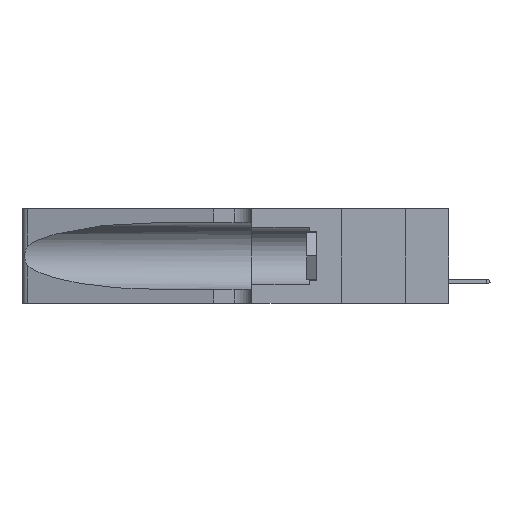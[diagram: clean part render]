
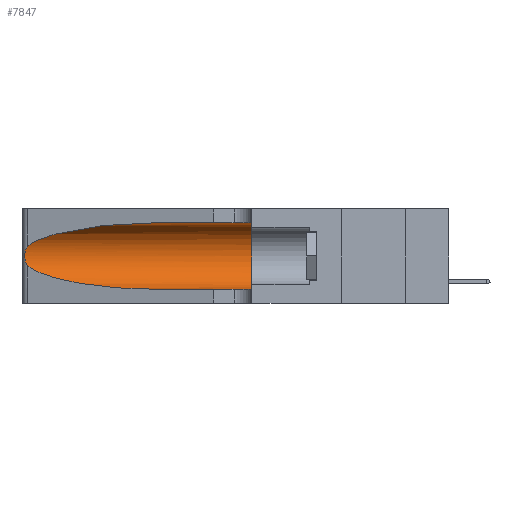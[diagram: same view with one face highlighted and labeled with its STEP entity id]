
A CAD part, left-side view. The second image highlights one B-rep face of the part: STEP entity #7847.
In plain terms, the highlighted cylindrical face has radius 3.308 mm (diameter 6.617 mm), a partial arc.
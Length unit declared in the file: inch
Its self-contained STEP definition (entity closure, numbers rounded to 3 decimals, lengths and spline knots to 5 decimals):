
#718 = LINE ( 'NONE', #38423, #27202 ) ;
#2604 = B_SPLINE_CURVE_WITH_KNOTS ( 'NONE', 3,
 ( #21177, #10785, #30940, #25056, #38808, #35554, #11384, #17910, #32139, #31533, #13188, #12435, #8761, #18988 ),
 .UNSPECIFIED., .F., .F.,
 ( 4, 2, 2, 2, 2, 2, 4 ),
 ( 0., 0.00027, 0.00053, 0.00107, 0.0016, 0.00187, 0.00214 ),
 .UNSPECIFIED. ) ;
#3382 = LINE ( 'NONE', #12412, #14491 ) ;
#3507 = CIRCLE ( 'NONE', #7570, 0.13025 ) ;
#3536 = DIRECTION ( 'NONE',  ( 0., 0., -1. ) ) ;
#4302 = CARTESIAN_POINT ( 'NONE',  ( 0.1305, 0.35, 0.185 ) ) ;
#5955 = CYLINDRICAL_SURFACE ( 'NONE', #28047, 0.13025 ) ;
#7346 = CARTESIAN_POINT ( 'NONE',  ( 0.25487, 1.22718, 0.22369 ) ) ;
#7570 = AXIS2_PLACEMENT_3D ( 'NONE', #4302, #42132, #24488 ) ;
#7847 = ADVANCED_FACE ( 'NONE', ( #40382 ), #5955, .F. ) ;
#8421 = CARTESIAN_POINT ( 'NONE',  ( 0.18966, 0.96281, 0.05475 ) ) ;
#8761 = CARTESIAN_POINT ( 'NONE',  ( 0.25555, 1.22993, 0.14849 ) ) ;
#10785 = CARTESIAN_POINT ( 'NONE',  ( 0.25555, 1.22994, 0.2215 ) ) ;
#11384 = CARTESIAN_POINT ( 'NONE',  ( 0.26075, 1.23896, 0.19203 ) ) ;
#12203 = VERTEX_POINT ( 'NONE', #19105 ) ;
#12210 = EDGE_CURVE ( 'NONE', #22186, #27137, #3382, .T. ) ;
#12412 = CARTESIAN_POINT ( 'NONE',  ( 0.1305, 1.61858, 0.31525 ) ) ;
#12435 = CARTESIAN_POINT ( 'NONE',  ( 0.25639, 1.23186, 0.15144 ) ) ;
#12762 = CARTESIAN_POINT ( 'NONE',  ( 0.1305, 1.61858, 0.185 ) ) ;
#13188 = CARTESIAN_POINT ( 'NONE',  ( 0.25789, 1.23486, 0.15765 ) ) ;
#13807 = EDGE_CURVE ( 'NONE', #12203, #26844, #2604, .T. ) ;
#14491 = VECTOR ( 'NONE', #35520, 39.37008 ) ;
#14600 = CARTESIAN_POINT ( 'NONE',  ( 0.2373, 1.15595, 0.28018 ) ) ;
#15310 =( BOUNDED_CURVE ( )  B_SPLINE_CURVE ( 3, ( #24737, #34623, #14600, #7346 ),
 .UNSPECIFIED., .F., .F. ) 
 B_SPLINE_CURVE_WITH_KNOTS ( ( 4, 4 ),
 ( 1.5708, 2.84003 ),
 .UNSPECIFIED. ) 
 CURVE ( )  GEOMETRIC_REPRESENTATION_ITEM ( )  RATIONAL_B_SPLINE_CURVE ( ( 1., 0.87, 0.87, 1. ) ) 
 REPRESENTATION_ITEM ( '' )  );
#16013 = VERTEX_POINT ( 'NONE', #42898 ) ;
#16032 = EDGE_LOOP ( 'NONE', ( #30787, #27376, #26366, #33218, #40699, #40232 ) ) ;
#17910 = CARTESIAN_POINT ( 'NONE',  ( 0.26075, 1.23896, 0.178 ) ) ;
#18988 = CARTESIAN_POINT ( 'NONE',  ( 0.25487, 1.22718, 0.14631 ) ) ;
#19105 = CARTESIAN_POINT ( 'NONE',  ( 0.25487, 1.22718, 0.22369 ) ) ;
#21177 = CARTESIAN_POINT ( 'NONE',  ( 0.25487, 1.22718, 0.22369 ) ) ;
#21253 = CARTESIAN_POINT ( 'NONE',  ( 0.25487, 1.22718, 0.14631 ) ) ;
#21628 = CARTESIAN_POINT ( 'NONE',  ( 0.1305, 0.35, 0.31525 ) ) ;
#22062 = CARTESIAN_POINT ( 'NONE',  ( 0.1305, 0.72297, 0.05475 ) ) ;
#22181 = DIRECTION ( 'NONE',  ( 0., -1., 0. ) ) ;
#22186 = VERTEX_POINT ( 'NONE', #26399 ) ;
#22214 = CARTESIAN_POINT ( 'NONE',  ( 0.2373, 1.15595, 0.08982 ) ) ;
#23741 =( BOUNDED_CURVE ( )  B_SPLINE_CURVE ( 3, ( #32578, #22214, #8421, #22062 ),
 .UNSPECIFIED., .F., .F. ) 
 B_SPLINE_CURVE_WITH_KNOTS ( ( 4, 4 ),
 ( 3.44316, 4.71239 ),
 .UNSPECIFIED. ) 
 CURVE ( )  GEOMETRIC_REPRESENTATION_ITEM ( )  RATIONAL_B_SPLINE_CURVE ( ( 1., 0.87, 0.87, 1. ) ) 
 REPRESENTATION_ITEM ( '' )  );
#24488 = DIRECTION ( 'NONE',  ( 0., 0., 1. ) ) ;
#24737 = CARTESIAN_POINT ( 'NONE',  ( 0.1305, 0.72297, 0.31525 ) ) ;
#25056 = CARTESIAN_POINT ( 'NONE',  ( 0.25787, 1.23484, 0.2124 ) ) ;
#26005 = DIRECTION ( 'NONE',  ( 0., -1., 0. ) ) ;
#26366 = ORIENTED_EDGE ( 'NONE', *, *, #28418, .T. ) ;
#26399 = CARTESIAN_POINT ( 'NONE',  ( 0.1305, 0.72297, 0.31525 ) ) ;
#26844 = VERTEX_POINT ( 'NONE', #21253 ) ;
#27137 = VERTEX_POINT ( 'NONE', #21628 ) ;
#27202 = VECTOR ( 'NONE', #22181, 39.37008 ) ;
#27376 = ORIENTED_EDGE ( 'NONE', *, *, #13807, .T. ) ;
#28047 = AXIS2_PLACEMENT_3D ( 'NONE', #12762, #26005, #3536 ) ;
#28418 = EDGE_CURVE ( 'NONE', #26844, #28620, #23741, .T. ) ;
#28620 = VERTEX_POINT ( 'NONE', #38870 ) ;
#30249 = EDGE_CURVE ( 'NONE', #28620, #16013, #718, .T. ) ;
#30787 = ORIENTED_EDGE ( 'NONE', *, *, #34459, .T. ) ;
#30940 = CARTESIAN_POINT ( 'NONE',  ( 0.25639, 1.23184, 0.21858 ) ) ;
#31533 = CARTESIAN_POINT ( 'NONE',  ( 0.25856, 1.23593, 0.16098 ) ) ;
#32139 = CARTESIAN_POINT ( 'NONE',  ( 0.26017, 1.23833, 0.17102 ) ) ;
#32578 = CARTESIAN_POINT ( 'NONE',  ( 0.25487, 1.22718, 0.14631 ) ) ;
#33218 = ORIENTED_EDGE ( 'NONE', *, *, #30249, .T. ) ;
#33864 = EDGE_CURVE ( 'NONE', #27137, #16013, #3507, .T. ) ;
#34459 = EDGE_CURVE ( 'NONE', #22186, #12203, #15310, .T. ) ;
#34623 = CARTESIAN_POINT ( 'NONE',  ( 0.18966, 0.96281, 0.31525 ) ) ;
#35520 = DIRECTION ( 'NONE',  ( 0., -1., 0. ) ) ;
#35554 = CARTESIAN_POINT ( 'NONE',  ( 0.26018, 1.23835, 0.19895 ) ) ;
#38423 = CARTESIAN_POINT ( 'NONE',  ( 0.1305, 1.61858, 0.05475 ) ) ;
#38808 = CARTESIAN_POINT ( 'NONE',  ( 0.25854, 1.2359, 0.20912 ) ) ;
#38870 = CARTESIAN_POINT ( 'NONE',  ( 0.1305, 0.72297, 0.05475 ) ) ;
#40232 = ORIENTED_EDGE ( 'NONE', *, *, #12210, .F. ) ;
#40382 = FACE_OUTER_BOUND ( 'NONE', #16032, .T. ) ;
#40699 = ORIENTED_EDGE ( 'NONE', *, *, #33864, .F. ) ;
#42132 = DIRECTION ( 'NONE',  ( 0., 1., 0. ) ) ;
#42898 = CARTESIAN_POINT ( 'NONE',  ( 0.1305, 0.35, 0.05475 ) ) ;
